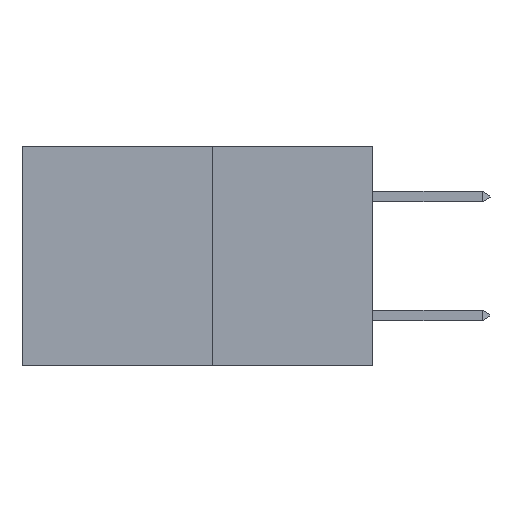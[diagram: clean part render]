
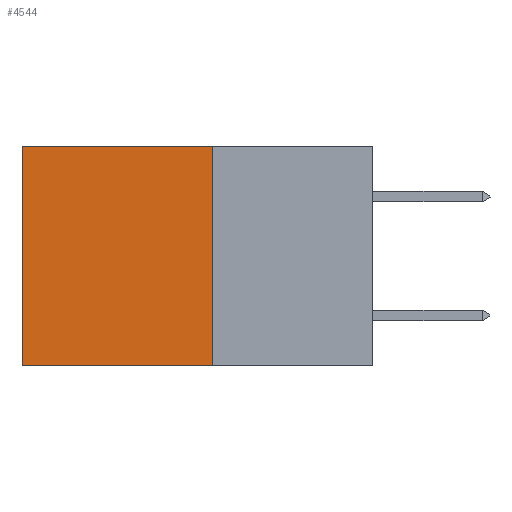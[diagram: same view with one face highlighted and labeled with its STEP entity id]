
A CAD part, left-side view. The second image highlights one B-rep face of the part: STEP entity #4544.
In plain terms, the highlighted planar face has unit normal (-1, 0, 0).
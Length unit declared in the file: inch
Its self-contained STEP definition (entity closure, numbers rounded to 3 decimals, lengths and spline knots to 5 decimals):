
#497 = CARTESIAN_POINT ( 'NONE',  ( 0.277, 0.27, -0.37 ) ) ;
#563 = DIRECTION ( 'NONE',  ( 0., 0., -1. ) ) ;
#566 = EDGE_CURVE ( 'NONE', #13303, #16993, #11431, .T. ) ;
#686 = CARTESIAN_POINT ( 'NONE',  ( 0.277, 0.59, -0.37 ) ) ;
#848 = ORIENTED_EDGE ( 'NONE', *, *, #9356, .F. ) ;
#1053 = DIRECTION ( 'NONE',  ( 0., 0., -1. ) ) ;
#1630 = DIRECTION ( 'NONE',  ( 1., 0., 0. ) ) ;
#1653 = EDGE_LOOP ( 'NONE', ( #9775, #9995, #848, #12357 ) ) ;
#2437 = LINE ( 'NONE', #497, #17385 ) ;
#2446 = CARTESIAN_POINT ( 'NONE',  ( 0.277, 0.27, 0. ) ) ;
#2606 = CARTESIAN_POINT ( 'NONE',  ( 0.277, 0.27, 0. ) ) ;
#2710 = EDGE_CURVE ( 'NONE', #2788, #16993, #16785, .T. ) ;
#2788 = VERTEX_POINT ( 'NONE', #13676 ) ;
#3082 = CARTESIAN_POINT ( 'NONE',  ( 0.277, 0.27, -0.37 ) ) ;
#4403 = LINE ( 'NONE', #2606, #8396 ) ;
#4544 = ADVANCED_FACE ( 'NONE', ( #18910 ), #15574, .F. ) ;
#5580 = DIRECTION ( 'NONE',  ( 0., 1., 0. ) ) ;
#7375 = VECTOR ( 'NONE', #9733, 39.37008 ) ;
#8105 = VERTEX_POINT ( 'NONE', #2446 ) ;
#8161 = CARTESIAN_POINT ( 'NONE',  ( 0.277, 0.59, -0.37 ) ) ;
#8396 = VECTOR ( 'NONE', #5580, 39.37008 ) ;
#9356 = EDGE_CURVE ( 'NONE', #8105, #2788, #2437, .T. ) ;
#9733 = DIRECTION ( 'NONE',  ( 0., 0., -1. ) ) ;
#9775 = ORIENTED_EDGE ( 'NONE', *, *, #566, .T. ) ;
#9995 = ORIENTED_EDGE ( 'NONE', *, *, #2710, .F. ) ;
#11431 = LINE ( 'NONE', #686, #7375 ) ;
#12357 = ORIENTED_EDGE ( 'NONE', *, *, #13707, .T. ) ;
#12997 = VECTOR ( 'NONE', #18122, 39.37008 ) ;
#13303 = VERTEX_POINT ( 'NONE', #16609 ) ;
#13676 = CARTESIAN_POINT ( 'NONE',  ( 0.277, 0.27, -0.37 ) ) ;
#13707 = EDGE_CURVE ( 'NONE', #8105, #13303, #4403, .T. ) ;
#14868 = CARTESIAN_POINT ( 'NONE',  ( 0.277, 0.27, -0.37 ) ) ;
#15574 = PLANE ( 'NONE',  #16961 ) ;
#16609 = CARTESIAN_POINT ( 'NONE',  ( 0.277, 0.59, 0. ) ) ;
#16785 = LINE ( 'NONE', #14868, #12997 ) ;
#16961 = AXIS2_PLACEMENT_3D ( 'NONE', #3082, #1630, #1053 ) ;
#16993 = VERTEX_POINT ( 'NONE', #8161 ) ;
#17385 = VECTOR ( 'NONE', #563, 39.37008 ) ;
#18122 = DIRECTION ( 'NONE',  ( 0., 1., 0. ) ) ;
#18910 = FACE_OUTER_BOUND ( 'NONE', #1653, .T. ) ;
